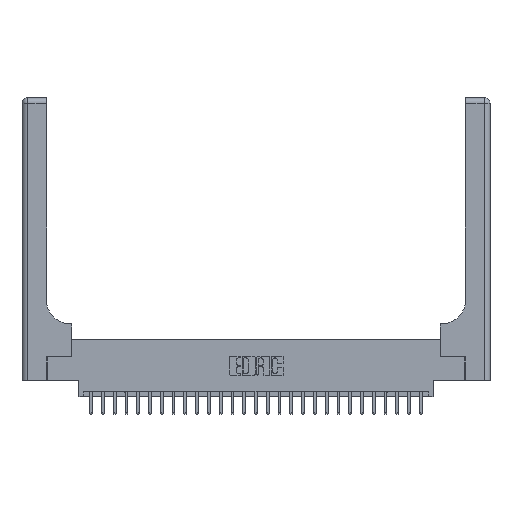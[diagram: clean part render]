
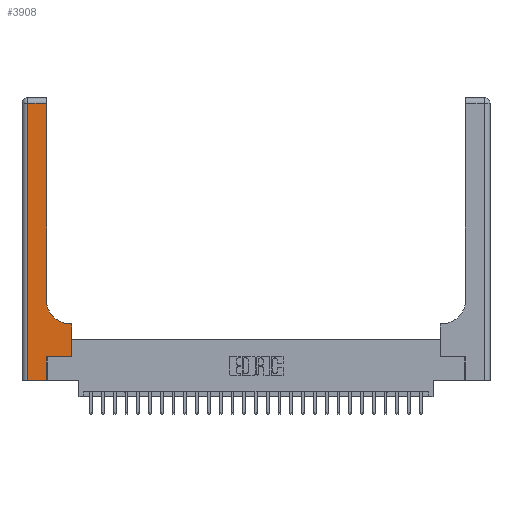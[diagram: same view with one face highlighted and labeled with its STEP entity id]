
A CAD part, top view. The second image highlights one B-rep face of the part: STEP entity #3908.
In plain terms, the highlighted planar face has unit normal (0, 0, 1).
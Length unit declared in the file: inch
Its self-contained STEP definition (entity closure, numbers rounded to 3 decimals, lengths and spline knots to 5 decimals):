
#528 = CARTESIAN_POINT ( 'NONE',  ( 0.26, 0.6, 0.37 ) ) ;
#571 = CARTESIAN_POINT ( 'NONE',  ( 0.06, 3., 0.37 ) ) ;
#765 = ORIENTED_EDGE ( 'NONE', *, *, #2728, .T. ) ;
#995 = VECTOR ( 'NONE', #22648, 39.37008 ) ;
#2728 = EDGE_CURVE ( 'NONE', #19661, #6603, #13296, .T. ) ;
#2836 = CARTESIAN_POINT ( 'NONE',  ( 0.265, 0.25, 0.37 ) ) ;
#2949 = EDGE_CURVE ( 'NONE', #6603, #11005, #19583, .T. ) ;
#3145 = ORIENTED_EDGE ( 'NONE', *, *, #19206, .T. ) ;
#3908 = ADVANCED_FACE ( 'NONE', ( #8249 ), #6536, .F. ) ;
#4492 = ORIENTED_EDGE ( 'NONE', *, *, #24477, .T. ) ;
#4787 = LINE ( 'NONE', #17780, #25545 ) ;
#4865 = EDGE_LOOP ( 'NONE', ( #22692, #7198, #18924, #23125, #3145, #14463, #4492, #6822, #765 ) ) ;
#4931 = VERTEX_POINT ( 'NONE', #2836 ) ;
#5081 = CARTESIAN_POINT ( 'NONE',  ( 0.51, 0.6, 0.37 ) ) ;
#5201 = LINE ( 'NONE', #8587, #995 ) ;
#5302 = DIRECTION ( 'NONE',  ( 1., 0., 0. ) ) ;
#5540 = DIRECTION ( 'NONE',  ( -1., 0., 0. ) ) ;
#5603 = DIRECTION ( 'NONE',  ( 0., 0., -1. ) ) ;
#5637 = CARTESIAN_POINT ( 'NONE',  ( 0., 3., 0.37 ) ) ;
#6449 = CARTESIAN_POINT ( 'NONE',  ( 0.26, 0.85, 0.37 ) ) ;
#6536 = PLANE ( 'NONE',  #13785 ) ;
#6556 = DIRECTION ( 'NONE',  ( 1., 0., 0. ) ) ;
#6603 = VERTEX_POINT ( 'NONE', #6449 ) ;
#6822 = ORIENTED_EDGE ( 'NONE', *, *, #9642, .T. ) ;
#6837 = DIRECTION ( 'NONE',  ( 0., 0., -1. ) ) ;
#6931 = CARTESIAN_POINT ( 'NONE',  ( 0.51, 0.85, 0.37 ) ) ;
#7198 = ORIENTED_EDGE ( 'NONE', *, *, #7999, .T. ) ;
#7887 = DIRECTION ( 'NONE',  ( 0., 1., 0. ) ) ;
#7999 = EDGE_CURVE ( 'NONE', #11005, #21529, #8412, .T. ) ;
#8249 = FACE_OUTER_BOUND ( 'NONE', #4865, .T. ) ;
#8412 = LINE ( 'NONE', #23799, #23788 ) ;
#8587 = CARTESIAN_POINT ( 'NONE',  ( 0., 0., 0.37 ) ) ;
#8769 = VECTOR ( 'NONE', #8849, 39.37008 ) ;
#8849 = DIRECTION ( 'NONE',  ( 0., -1., 0. ) ) ;
#9624 = VECTOR ( 'NONE', #18795, 39.37008 ) ;
#9642 = EDGE_CURVE ( 'NONE', #9775, #19661, #10231, .T. ) ;
#9675 = LINE ( 'NONE', #23309, #20974 ) ;
#9775 = VERTEX_POINT ( 'NONE', #17124 ) ;
#10231 = LINE ( 'NONE', #528, #9624 ) ;
#10745 = LINE ( 'NONE', #19384, #16088 ) ;
#11005 = VERTEX_POINT ( 'NONE', #12791 ) ;
#11196 = VERTEX_POINT ( 'NONE', #23343 ) ;
#12437 = EDGE_CURVE ( 'NONE', #4931, #24914, #10745, .T. ) ;
#12791 = CARTESIAN_POINT ( 'NONE',  ( 0.26, 2.94, 0.37 ) ) ;
#13296 = CIRCLE ( 'NONE', #16637, 0.25 ) ;
#13785 = AXIS2_PLACEMENT_3D ( 'NONE', #5637, #5603, #5540 ) ;
#14463 = ORIENTED_EDGE ( 'NONE', *, *, #12437, .T. ) ;
#14699 = LINE ( 'NONE', #571, #8769 ) ;
#14866 = VECTOR ( 'NONE', #23919, 39.37008 ) ;
#15055 = CARTESIAN_POINT ( 'NONE',  ( 0.06, 2.94, 0.37 ) ) ;
#15307 = EDGE_CURVE ( 'NONE', #20235, #11196, #5201, .T. ) ;
#16088 = VECTOR ( 'NONE', #5302, 39.37008 ) ;
#16506 = CARTESIAN_POINT ( 'NONE',  ( 0.528, 0.25, 0.37 ) ) ;
#16637 = AXIS2_PLACEMENT_3D ( 'NONE', #6931, #6837, #6556 ) ;
#17124 = CARTESIAN_POINT ( 'NONE',  ( 0.528, 0.6, 0.37 ) ) ;
#17780 = CARTESIAN_POINT ( 'NONE',  ( 0.265, 0., 0.37 ) ) ;
#18795 = DIRECTION ( 'NONE',  ( -1., 0., 0. ) ) ;
#18924 = ORIENTED_EDGE ( 'NONE', *, *, #23835, .T. ) ;
#19206 = EDGE_CURVE ( 'NONE', #11196, #4931, #4787, .T. ) ;
#19324 = DIRECTION ( 'NONE',  ( 0., 1., 0. ) ) ;
#19384 = CARTESIAN_POINT ( 'NONE',  ( 0.265, 0.25, 0.37 ) ) ;
#19583 = LINE ( 'NONE', #24000, #14866 ) ;
#19661 = VERTEX_POINT ( 'NONE', #5081 ) ;
#20235 = VERTEX_POINT ( 'NONE', #23308 ) ;
#20974 = VECTOR ( 'NONE', #19324, 39.37008 ) ;
#21529 = VERTEX_POINT ( 'NONE', #15055 ) ;
#21799 = DIRECTION ( 'NONE',  ( -1., 0., 0. ) ) ;
#22648 = DIRECTION ( 'NONE',  ( 1., 0., 0. ) ) ;
#22692 = ORIENTED_EDGE ( 'NONE', *, *, #2949, .T. ) ;
#23125 = ORIENTED_EDGE ( 'NONE', *, *, #15307, .T. ) ;
#23308 = CARTESIAN_POINT ( 'NONE',  ( 0.06, 0., 0.37 ) ) ;
#23309 = CARTESIAN_POINT ( 'NONE',  ( 0.528, 0.25, 0.37 ) ) ;
#23343 = CARTESIAN_POINT ( 'NONE',  ( 0.265, 0., 0.37 ) ) ;
#23788 = VECTOR ( 'NONE', #21799, 39.37008 ) ;
#23799 = CARTESIAN_POINT ( 'NONE',  ( 0., 2.94, 0.37 ) ) ;
#23835 = EDGE_CURVE ( 'NONE', #21529, #20235, #14699, .T. ) ;
#23919 = DIRECTION ( 'NONE',  ( 0., 1., 0. ) ) ;
#24000 = CARTESIAN_POINT ( 'NONE',  ( 0.26, 3., 0.37 ) ) ;
#24477 = EDGE_CURVE ( 'NONE', #24914, #9775, #9675, .T. ) ;
#24914 = VERTEX_POINT ( 'NONE', #16506 ) ;
#25545 = VECTOR ( 'NONE', #7887, 39.37008 ) ;
